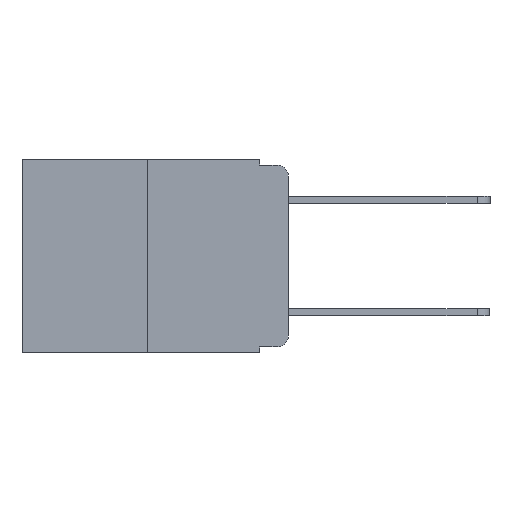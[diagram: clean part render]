
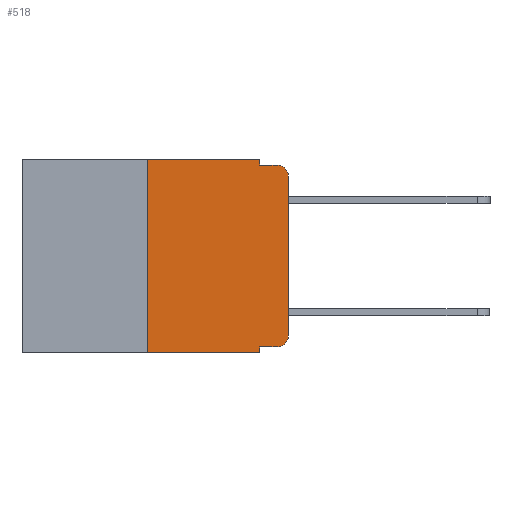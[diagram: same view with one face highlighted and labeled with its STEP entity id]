
A CAD part, left-side view. The second image highlights one B-rep face of the part: STEP entity #518.
In plain terms, the highlighted planar face has unit normal (-1, 0, 0).
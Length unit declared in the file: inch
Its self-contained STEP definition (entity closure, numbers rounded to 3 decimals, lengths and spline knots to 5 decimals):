
#127 = DIRECTION ( 'NONE',  ( 0., -1., 0. ) ) ;
#128 = LINE ( 'NONE', #6932, #4553 ) ;
#325 = CARTESIAN_POINT ( 'NONE',  ( 0., 0.051, 0. ) ) ;
#448 = FACE_OUTER_BOUND ( 'NONE', #8498, .T. ) ;
#506 = DIRECTION ( 'NONE',  ( 0., -1., 0. ) ) ;
#518 = ADVANCED_FACE ( 'NONE', ( #448 ), #2509, .F. ) ;
#577 = CARTESIAN_POINT ( 'NONE',  ( 0., 0., -0.313 ) ) ;
#602 = ORIENTED_EDGE ( 'NONE', *, *, #7769, .T. ) ;
#616 = ORIENTED_EDGE ( 'NONE', *, *, #9862, .F. ) ;
#770 = AXIS2_PLACEMENT_3D ( 'NONE', #3587, #9328, #4532 ) ;
#900 = VERTEX_POINT ( 'NONE', #577 ) ;
#1014 = VERTEX_POINT ( 'NONE', #10991 ) ;
#1125 = EDGE_CURVE ( 'NONE', #1014, #3272, #1340, .T. ) ;
#1340 = LINE ( 'NONE', #325, #10059 ) ;
#1391 = CARTESIAN_POINT ( 'NONE',  ( 0., 0.25, 0. ) ) ;
#1407 = DIRECTION ( 'NONE',  ( 0., 0., -1. ) ) ;
#1815 = ORIENTED_EDGE ( 'NONE', *, *, #4286, .T. ) ;
#1875 = CARTESIAN_POINT ( 'NONE',  ( 0., 0.473, 0. ) ) ;
#1900 = EDGE_CURVE ( 'NONE', #2552, #1014, #8693, .T. ) ;
#1907 = VECTOR ( 'NONE', #506, 39.37008 ) ;
#2342 = LINE ( 'NONE', #7401, #8819 ) ;
#2422 = CARTESIAN_POINT ( 'NONE',  ( 0., 0.02, -0.03 ) ) ;
#2509 = PLANE ( 'NONE',  #7432 ) ;
#2552 = VERTEX_POINT ( 'NONE', #1391 ) ;
#2749 = DIRECTION ( 'NONE',  ( 1., 0., 0. ) ) ;
#2794 = CARTESIAN_POINT ( 'NONE',  ( 0., 0.473, 0. ) ) ;
#2853 = DIRECTION ( 'NONE',  ( 0., -1., 0. ) ) ;
#3000 = EDGE_CURVE ( 'NONE', #3272, #7701, #9771, .T. ) ;
#3272 = VERTEX_POINT ( 'NONE', #8867 ) ;
#3587 = CARTESIAN_POINT ( 'NONE',  ( 0., 0.02, -0.313 ) ) ;
#3672 = CARTESIAN_POINT ( 'NONE',  ( 0., 0.051, -0.343 ) ) ;
#4052 = CARTESIAN_POINT ( 'NONE',  ( 0., 0.25, -0.343 ) ) ;
#4066 = VECTOR ( 'NONE', #7698, 39.37008 ) ;
#4274 = VERTEX_POINT ( 'NONE', #4052 ) ;
#4286 = EDGE_CURVE ( 'NONE', #5122, #7701, #6468, .T. ) ;
#4332 = CARTESIAN_POINT ( 'NONE',  ( 0., 0., -0.03 ) ) ;
#4456 = ORIENTED_EDGE ( 'NONE', *, *, #9344, .T. ) ;
#4532 = DIRECTION ( 'NONE',  ( 0., 0., -1. ) ) ;
#4553 = VECTOR ( 'NONE', #8514, 39.37008 ) ;
#4673 = VECTOR ( 'NONE', #2853, 39.37008 ) ;
#4702 = ORIENTED_EDGE ( 'NONE', *, *, #1125, .F. ) ;
#4757 = AXIS2_PLACEMENT_3D ( 'NONE', #2422, #8258, #5348 ) ;
#4858 = ORIENTED_EDGE ( 'NONE', *, *, #3000, .F. ) ;
#4926 = DIRECTION ( 'NONE',  ( 0., -1., 0. ) ) ;
#4972 = VERTEX_POINT ( 'NONE', #7154 ) ;
#5008 = CARTESIAN_POINT ( 'NONE',  ( 0., 0.051, -0.01 ) ) ;
#5122 = VERTEX_POINT ( 'NONE', #4332 ) ;
#5210 = VECTOR ( 'NONE', #4926, 39.37008 ) ;
#5228 = CARTESIAN_POINT ( 'NONE',  ( 0., 0.02, -0.01 ) ) ;
#5233 = CARTESIAN_POINT ( 'NONE',  ( 0., 0., 0. ) ) ;
#5348 = DIRECTION ( 'NONE',  ( 0., 0., -1. ) ) ;
#5428 = EDGE_CURVE ( 'NONE', #900, #5122, #8412, .T. ) ;
#5532 = CARTESIAN_POINT ( 'NONE',  ( 0., 0.051, -0.333 ) ) ;
#5747 = VERTEX_POINT ( 'NONE', #5532 ) ;
#6270 = CIRCLE ( 'NONE', #770, 0.02 ) ;
#6468 = CIRCLE ( 'NONE', #4757, 0.02 ) ;
#6854 = LINE ( 'NONE', #10315, #4673 ) ;
#6932 = CARTESIAN_POINT ( 'NONE',  ( 0., 0.051, 0. ) ) ;
#7154 = CARTESIAN_POINT ( 'NONE',  ( 0., 0.02, -0.333 ) ) ;
#7401 = CARTESIAN_POINT ( 'NONE',  ( 0., 0.25, 0. ) ) ;
#7432 = AXIS2_PLACEMENT_3D ( 'NONE', #2794, #2749, #1407 ) ;
#7502 = ORIENTED_EDGE ( 'NONE', *, *, #10956, .F. ) ;
#7604 = LINE ( 'NONE', #8893, #5210 ) ;
#7698 = DIRECTION ( 'NONE',  ( 0., 0., 1. ) ) ;
#7701 = VERTEX_POINT ( 'NONE', #5228 ) ;
#7769 = EDGE_CURVE ( 'NONE', #4972, #900, #6270, .T. ) ;
#8258 = DIRECTION ( 'NONE',  ( -1., 0., 0. ) ) ;
#8412 = LINE ( 'NONE', #5233, #4066 ) ;
#8498 = EDGE_LOOP ( 'NONE', ( #8621, #1815, #4858, #4702, #9701, #7502, #8500, #616, #4456, #602 ) ) ;
#8500 = ORIENTED_EDGE ( 'NONE', *, *, #8888, .T. ) ;
#8514 = DIRECTION ( 'NONE',  ( 0., 0., -1. ) ) ;
#8621 = ORIENTED_EDGE ( 'NONE', *, *, #5428, .T. ) ;
#8693 = LINE ( 'NONE', #1875, #1907 ) ;
#8819 = VECTOR ( 'NONE', #10529, 39.37008 ) ;
#8867 = CARTESIAN_POINT ( 'NONE',  ( 0., 0.051, -0.01 ) ) ;
#8888 = EDGE_CURVE ( 'NONE', #4274, #9985, #7604, .T. ) ;
#8893 = CARTESIAN_POINT ( 'NONE',  ( 0., 0.473, -0.343 ) ) ;
#9328 = DIRECTION ( 'NONE',  ( -1., 0., 0. ) ) ;
#9344 = EDGE_CURVE ( 'NONE', #5747, #4972, #6854, .T. ) ;
#9701 = ORIENTED_EDGE ( 'NONE', *, *, #1900, .F. ) ;
#9771 = LINE ( 'NONE', #5008, #10288 ) ;
#9862 = EDGE_CURVE ( 'NONE', #5747, #9985, #128, .T. ) ;
#9985 = VERTEX_POINT ( 'NONE', #3672 ) ;
#10059 = VECTOR ( 'NONE', #10131, 39.37008 ) ;
#10131 = DIRECTION ( 'NONE',  ( 0., 0., -1. ) ) ;
#10288 = VECTOR ( 'NONE', #127, 39.37008 ) ;
#10315 = CARTESIAN_POINT ( 'NONE',  ( 0., 0.051, -0.333 ) ) ;
#10529 = DIRECTION ( 'NONE',  ( 0., 0., 1. ) ) ;
#10956 = EDGE_CURVE ( 'NONE', #4274, #2552, #2342, .T. ) ;
#10991 = CARTESIAN_POINT ( 'NONE',  ( 0., 0.051, 0. ) ) ;
